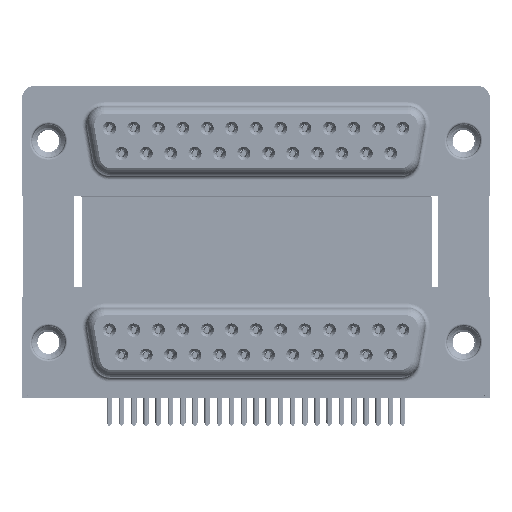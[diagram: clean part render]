
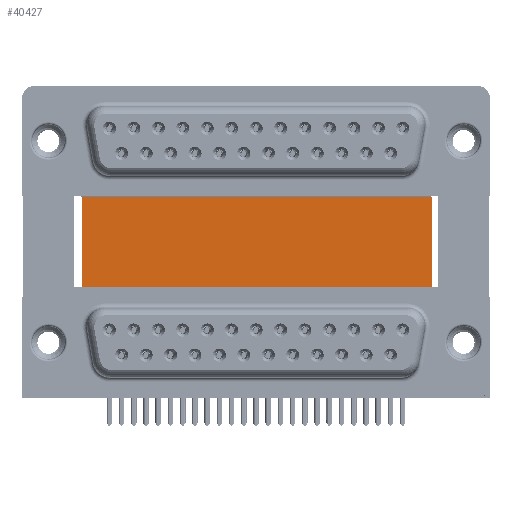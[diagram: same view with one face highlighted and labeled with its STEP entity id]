
A CAD part, top view. The second image highlights one B-rep face of the part: STEP entity #40427.
In plain terms, the highlighted planar face has unit normal (0, 0, 1).
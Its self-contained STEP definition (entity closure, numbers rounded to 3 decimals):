
#518 = CARTESIAN_POINT ( 'NONE',  ( 3.79, -3.735, -12. ) ) ;
#3078 = AXIS2_PLACEMENT_3D ( 'NONE', #38850, #20757, #20155 ) ;
#5438 = ORIENTED_EDGE ( 'NONE', *, *, #46031, .F. ) ;
#9425 = VERTEX_POINT ( 'NONE', #58224 ) ;
#11577 = FACE_OUTER_BOUND ( 'NONE', #14300, .T. ) ;
#13249 = CARTESIAN_POINT ( 'NONE',  ( 43.43, 16.585, -12. ) ) ;
#14300 = EDGE_LOOP ( 'NONE', ( #50415, #5438, #39285, #54003 ) ) ;
#14958 = EDGE_CURVE ( 'NONE', #18817, #41699, #58175, .T. ) ;
#16163 = PLANE ( 'NONE',  #3078 ) ;
#18817 = VERTEX_POINT ( 'NONE', #23608 ) ;
#20155 = DIRECTION ( 'NONE',  ( -1., 0., 0. ) ) ;
#20757 = DIRECTION ( 'NONE',  ( 0., 0., -1. ) ) ;
#21818 = VERTEX_POINT ( 'NONE', #47350 ) ;
#22272 = VECTOR ( 'NONE', #48985, 1000. ) ;
#23608 = CARTESIAN_POINT ( 'NONE',  ( 3.79, 16.585, -12. ) ) ;
#30348 = CARTESIAN_POINT ( 'NONE',  ( 3.79, 16.585, -12. ) ) ;
#32630 = VECTOR ( 'NONE', #36636, 1000. ) ;
#32721 = VECTOR ( 'NONE', #35931, 1000. ) ;
#33868 = LINE ( 'NONE', #518, #54361 ) ;
#33878 = EDGE_CURVE ( 'NONE', #18817, #21818, #40638, .T. ) ;
#34174 = DIRECTION ( 'NONE',  ( 1., 0., 0. ) ) ;
#35931 = DIRECTION ( 'NONE',  ( 0., -1., 0. ) ) ;
#36636 = DIRECTION ( 'NONE',  ( 1., 0., 0. ) ) ;
#36839 = LINE ( 'NONE', #13249, #32721 ) ;
#38850 = CARTESIAN_POINT ( 'NONE',  ( 3.79, 16.585, -12. ) ) ;
#39285 = ORIENTED_EDGE ( 'NONE', *, *, #33878, .F. ) ;
#40427 = ADVANCED_FACE ( 'NONE', ( #11577 ), #16163, .F. ) ;
#40638 = LINE ( 'NONE', #51314, #32630 ) ;
#41699 = VERTEX_POINT ( 'NONE', #58103 ) ;
#46031 = EDGE_CURVE ( 'NONE', #21818, #9425, #36839, .T. ) ;
#47350 = CARTESIAN_POINT ( 'NONE',  ( 43.43, 16.585, -12. ) ) ;
#48425 = EDGE_CURVE ( 'NONE', #41699, #9425, #33868, .T. ) ;
#48985 = DIRECTION ( 'NONE',  ( 0., -1., 0. ) ) ;
#50415 = ORIENTED_EDGE ( 'NONE', *, *, #48425, .T. ) ;
#51314 = CARTESIAN_POINT ( 'NONE',  ( 3.79, 16.585, -12. ) ) ;
#54003 = ORIENTED_EDGE ( 'NONE', *, *, #14958, .T. ) ;
#54361 = VECTOR ( 'NONE', #34174, 1000. ) ;
#58103 = CARTESIAN_POINT ( 'NONE',  ( 3.79, -3.735, -12. ) ) ;
#58175 = LINE ( 'NONE', #30348, #22272 ) ;
#58224 = CARTESIAN_POINT ( 'NONE',  ( 43.43, -3.735, -12. ) ) ;
